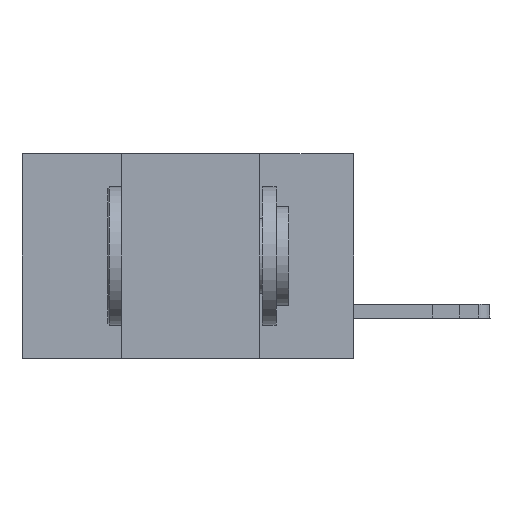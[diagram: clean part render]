
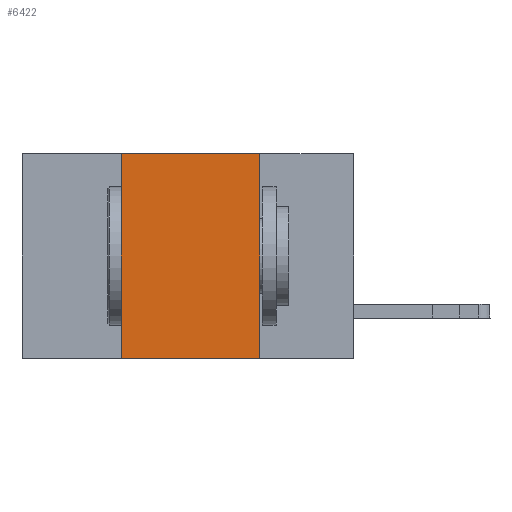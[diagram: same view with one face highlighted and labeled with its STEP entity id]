
A CAD part, left-side view. The second image highlights one B-rep face of the part: STEP entity #6422.
In plain terms, the highlighted planar face has unit normal (-1, 0, 0).
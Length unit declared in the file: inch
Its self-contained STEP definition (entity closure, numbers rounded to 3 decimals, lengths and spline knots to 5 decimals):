
#533 = VERTEX_POINT ( 'NONE', #15146 ) ;
#1325 = CARTESIAN_POINT ( 'NONE',  ( 0., 0.6, -0.37 ) ) ;
#2256 = AXIS2_PLACEMENT_3D ( 'NONE', #17655, #2971, #20139 ) ;
#2661 = VECTOR ( 'NONE', #16025, 39.37008 ) ;
#2971 = DIRECTION ( 'NONE',  ( 1., 0., 0. ) ) ;
#3546 = EDGE_LOOP ( 'NONE', ( #7817, #8574, #21675, #10125 ) ) ;
#3961 = VECTOR ( 'NONE', #16810, 39.37008 ) ;
#6422 = ADVANCED_FACE ( 'NONE', ( #9581 ), #29779, .F. ) ;
#7817 = ORIENTED_EDGE ( 'NONE', *, *, #29432, .F. ) ;
#8574 = ORIENTED_EDGE ( 'NONE', *, *, #14711, .F. ) ;
#8884 = VERTEX_POINT ( 'NONE', #22345 ) ;
#9581 = FACE_OUTER_BOUND ( 'NONE', #3546, .T. ) ;
#10002 = VECTOR ( 'NONE', #18471, 39.37008 ) ;
#10125 = ORIENTED_EDGE ( 'NONE', *, *, #15840, .T. ) ;
#10175 = VERTEX_POINT ( 'NONE', #12996 ) ;
#11046 = VECTOR ( 'NONE', #26213, 39.37008 ) ;
#12996 = CARTESIAN_POINT ( 'NONE',  ( 0., 0.17, -0.37 ) ) ;
#13565 = CARTESIAN_POINT ( 'NONE',  ( 0., 0.17, 0. ) ) ;
#14711 = EDGE_CURVE ( 'NONE', #8884, #533, #30064, .T. ) ;
#15146 = CARTESIAN_POINT ( 'NONE',  ( 0., 0.17, 0. ) ) ;
#15672 = LINE ( 'NONE', #13565, #2661 ) ;
#15840 = EDGE_CURVE ( 'NONE', #22670, #10175, #28824, .T. ) ;
#16025 = DIRECTION ( 'NONE',  ( 0., 0., -1. ) ) ;
#16810 = DIRECTION ( 'NONE',  ( 0., -1., 0. ) ) ;
#17581 = LINE ( 'NONE', #23783, #11046 ) ;
#17655 = CARTESIAN_POINT ( 'NONE',  ( 0., 0.6, 0. ) ) ;
#18471 = DIRECTION ( 'NONE',  ( 0., -1., 0. ) ) ;
#18494 = EDGE_CURVE ( 'NONE', #22670, #8884, #17581, .T. ) ;
#20139 = DIRECTION ( 'NONE',  ( 0., 0., -1. ) ) ;
#21675 = ORIENTED_EDGE ( 'NONE', *, *, #18494, .F. ) ;
#22345 = CARTESIAN_POINT ( 'NONE',  ( 0., 0.42, 0. ) ) ;
#22670 = VERTEX_POINT ( 'NONE', #27448 ) ;
#23783 = CARTESIAN_POINT ( 'NONE',  ( 0., 0.42, 0. ) ) ;
#26213 = DIRECTION ( 'NONE',  ( 0., 0., 1. ) ) ;
#27448 = CARTESIAN_POINT ( 'NONE',  ( 0., 0.42, -0.37 ) ) ;
#28824 = LINE ( 'NONE', #1325, #10002 ) ;
#29432 = EDGE_CURVE ( 'NONE', #533, #10175, #15672, .T. ) ;
#29779 = PLANE ( 'NONE',  #2256 ) ;
#30064 = LINE ( 'NONE', #31498, #3961 ) ;
#31498 = CARTESIAN_POINT ( 'NONE',  ( 0., 0.6, 0. ) ) ;
